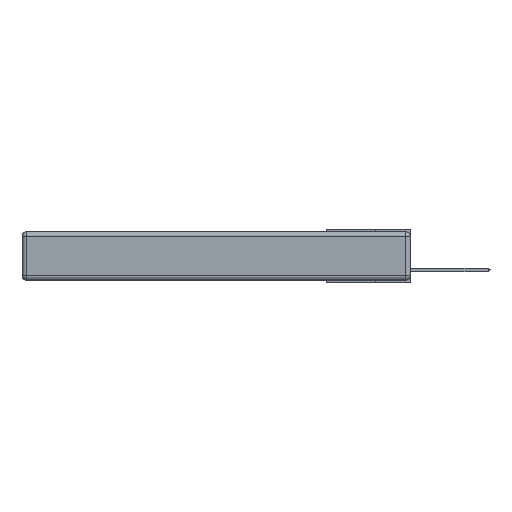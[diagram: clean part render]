
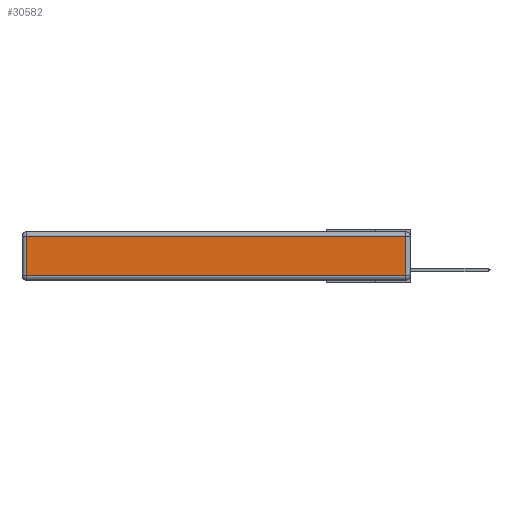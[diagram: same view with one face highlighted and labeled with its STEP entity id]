
A CAD part, left-side view. The second image highlights one B-rep face of the part: STEP entity #30582.
In plain terms, the highlighted planar face has unit normal (-1, 0, 0).
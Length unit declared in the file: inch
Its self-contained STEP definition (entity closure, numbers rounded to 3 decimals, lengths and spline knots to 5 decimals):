
#1770 = PLANE ( 'NONE',  #3983 ) ;
#3822 = CARTESIAN_POINT ( 'NONE',  ( 0., 2.72, -0.03 ) ) ;
#3983 = AXIS2_PLACEMENT_3D ( 'NONE', #23678, #8919, #23900 ) ;
#5345 = ORIENTED_EDGE ( 'NONE', *, *, #6409, .T. ) ;
#5667 = EDGE_CURVE ( 'NONE', #13818, #29822, #29322, .T. ) ;
#5758 = ORIENTED_EDGE ( 'NONE', *, *, #5667, .T. ) ;
#6320 = DIRECTION ( 'NONE',  ( 0., 1., 0. ) ) ;
#6409 = EDGE_CURVE ( 'NONE', #29822, #31605, #29266, .T. ) ;
#6440 = FACE_OUTER_BOUND ( 'NONE', #27487, .T. ) ;
#7562 = VECTOR ( 'NONE', #6320, 39.37008 ) ;
#7924 = ORIENTED_EDGE ( 'NONE', *, *, #19152, .T. ) ;
#8919 = DIRECTION ( 'NONE',  ( -1., 0., 0. ) ) ;
#10006 = DIRECTION ( 'NONE',  ( 0., -1., 0. ) ) ;
#10098 = CARTESIAN_POINT ( 'NONE',  ( 0., 2.72, -0.313 ) ) ;
#13102 = VECTOR ( 'NONE', #15217, 39.37008 ) ;
#13818 = VERTEX_POINT ( 'NONE', #30016 ) ;
#14766 = VECTOR ( 'NONE', #10006, 39.37008 ) ;
#15217 = DIRECTION ( 'NONE',  ( 0., 0., -1. ) ) ;
#16185 = ORIENTED_EDGE ( 'NONE', *, *, #25009, .T. ) ;
#19152 = EDGE_CURVE ( 'NONE', #20801, #13818, #20265, .T. ) ;
#19566 = CARTESIAN_POINT ( 'NONE',  ( 0., 0.03, -0.343 ) ) ;
#20265 = LINE ( 'NONE', #30033, #14766 ) ;
#20801 = VERTEX_POINT ( 'NONE', #10098 ) ;
#21402 = CARTESIAN_POINT ( 'NONE',  ( 0., 2.75, -0.03 ) ) ;
#22197 = CARTESIAN_POINT ( 'NONE',  ( 0., 2.72, -0.343 ) ) ;
#23678 = CARTESIAN_POINT ( 'NONE',  ( 0., 0., -0.343 ) ) ;
#23900 = DIRECTION ( 'NONE',  ( 0., 0., 1. ) ) ;
#25009 = EDGE_CURVE ( 'NONE', #31605, #20801, #27450, .T. ) ;
#25463 = VECTOR ( 'NONE', #29280, 39.37008 ) ;
#27450 = LINE ( 'NONE', #22197, #13102 ) ;
#27487 = EDGE_LOOP ( 'NONE', ( #7924, #5758, #5345, #16185 ) ) ;
#29266 = LINE ( 'NONE', #21402, #7562 ) ;
#29280 = DIRECTION ( 'NONE',  ( 0., 0., 1. ) ) ;
#29322 = LINE ( 'NONE', #19566, #25463 ) ;
#29822 = VERTEX_POINT ( 'NONE', #30140 ) ;
#30016 = CARTESIAN_POINT ( 'NONE',  ( 0., 0.03, -0.313 ) ) ;
#30033 = CARTESIAN_POINT ( 'NONE',  ( 0., 0., -0.313 ) ) ;
#30140 = CARTESIAN_POINT ( 'NONE',  ( 0., 0.03, -0.03 ) ) ;
#30582 = ADVANCED_FACE ( 'NONE', ( #6440 ), #1770, .T. ) ;
#31605 = VERTEX_POINT ( 'NONE', #3822 ) ;
